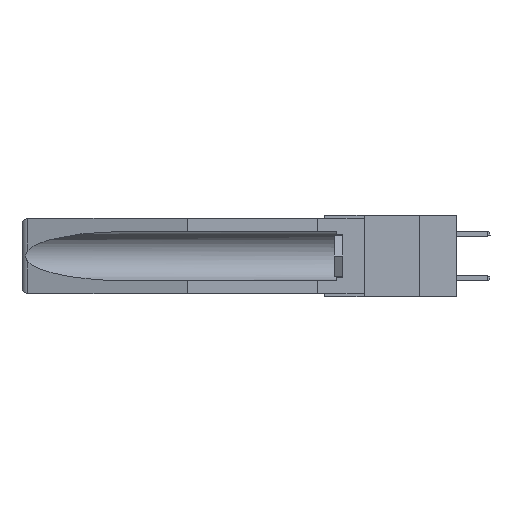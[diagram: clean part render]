
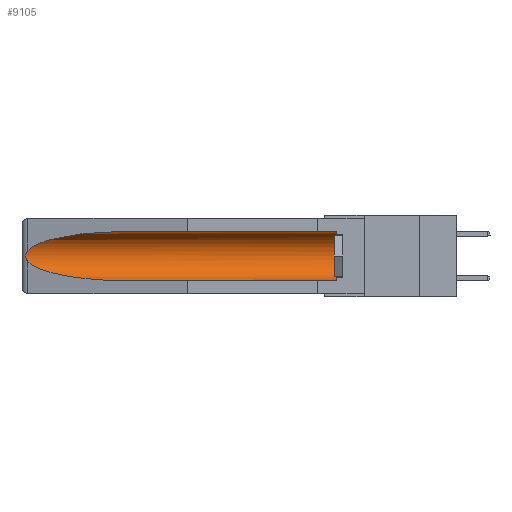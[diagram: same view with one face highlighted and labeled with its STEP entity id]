
A CAD part, left-side view. The second image highlights one B-rep face of the part: STEP entity #9105.
In plain terms, the highlighted cylindrical face has radius 2.857 mm (diameter 5.715 mm), a partial arc.
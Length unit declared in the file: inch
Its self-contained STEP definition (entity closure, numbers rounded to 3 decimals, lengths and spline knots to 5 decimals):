
#644 = DIRECTION ( 'NONE',  ( 0., 1., 0. ) ) ;
#1695 = VERTEX_POINT ( 'NONE', #3598 ) ;
#1882 = CARTESIAN_POINT ( 'NONE',  ( 0.155, 1.07973, -0.284 ) ) ;
#2290 = CARTESIAN_POINT ( 'NONE',  ( 0.155, -0.30754, -0.284 ) ) ;
#2295 = CIRCLE ( 'NONE', #18486, 0.1125 ) ;
#2348 = ORIENTED_EDGE ( 'NONE', *, *, #28603, .T. ) ;
#2690 = ORIENTED_EDGE ( 'NONE', *, *, #3187, .T. ) ;
#2977 = VECTOR ( 'NONE', #13010, 39.37008 ) ;
#3187 = EDGE_CURVE ( 'NONE', #1695, #21045, #13953, .T. ) ;
#3254 = CARTESIAN_POINT ( 'NONE',  ( 0.2673, 1.5327, -0.16383 ) ) ;
#3262 = AXIS2_PLACEMENT_3D ( 'NONE', #29101, #14131, #11287 ) ;
#3360 = CARTESIAN_POINT ( 'NONE',  ( 0.2675, 1.53308, -0.16763 ) ) ;
#3598 = CARTESIAN_POINT ( 'NONE',  ( 0.155, 1.07973, -0.059 ) ) ;
#4143 = CARTESIAN_POINT ( 'NONE',  ( 0.26537, 1.52718, -0.14972 ) ) ;
#5935 = CARTESIAN_POINT ( 'NONE',  ( 0.2675, 1.53308, -0.17534 ) ) ;
#7394 = CARTESIAN_POINT ( 'NONE',  ( 0.155, 0.126, -0.284 ) ) ;
#7539 = CARTESIAN_POINT ( 'NONE',  ( 0.21114, 1.30732, -0.284 ) ) ;
#8003 = CARTESIAN_POINT ( 'NONE',  ( 0.26537, 1.52718, -0.14972 ) ) ;
#8166 = CARTESIAN_POINT ( 'NONE',  ( 0.155, 0.126, -0.059 ) ) ;
#8216 = EDGE_CURVE ( 'NONE', #21045, #9767, #30933, .T. ) ;
#8225 = CARTESIAN_POINT ( 'NONE',  ( 0.26655, 1.53094, -0.18657 ) ) ;
#9105 = ADVANCED_FACE ( 'NONE', ( #24595 ), #30507, .F. ) ;
#9767 = VERTEX_POINT ( 'NONE', #27137 ) ;
#9859 = CARTESIAN_POINT ( 'NONE',  ( 0.25451, 1.48313, -0.24835 ) ) ;
#10286 = VERTEX_POINT ( 'NONE', #1882 ) ;
#10876 = ORIENTED_EDGE ( 'NONE', *, *, #23350, .T. ) ;
#11287 = DIRECTION ( 'NONE',  ( 0., 0., 1. ) ) ;
#11642 = ORIENTED_EDGE ( 'NONE', *, *, #8216, .T. ) ;
#12748 = DIRECTION ( 'NONE',  ( 0., -1., 0. ) ) ;
#12854 = CARTESIAN_POINT ( 'NONE',  ( 0.155, 0.126, -0.1715 ) ) ;
#13010 = DIRECTION ( 'NONE',  ( 0., 1., 0. ) ) ;
#13383 = CARTESIAN_POINT ( 'NONE',  ( 0.26537, 1.52718, -0.19328 ) ) ;
#13953 =( BOUNDED_CURVE ( )  B_SPLINE_CURVE ( 3, ( #27165, #21980, #19331, #19646 ),
 .UNSPECIFIED., .F., .F. ) 
 B_SPLINE_CURVE_WITH_KNOTS ( ( 4, 4 ),
 ( 4.71239, 6.08839 ),
 .UNSPECIFIED. ) 
 CURVE ( )  GEOMETRIC_REPRESENTATION_ITEM ( )  RATIONAL_B_SPLINE_CURVE ( ( 1., 0.848, 0.848, 1. ) ) 
 REPRESENTATION_ITEM ( '' )  );
#14131 = DIRECTION ( 'NONE',  ( 0., 1., 0. ) ) ;
#15490 = CARTESIAN_POINT ( 'NONE',  ( 0.26597, 1.52961, -0.15275 ) ) ;
#17339 = CARTESIAN_POINT ( 'NONE',  ( 0.26537, 1.52718, -0.19328 ) ) ;
#17913 = DIRECTION ( 'NONE',  ( 0., 0., 1. ) ) ;
#18486 = AXIS2_PLACEMENT_3D ( 'NONE', #12854, #12748, #17913 ) ;
#19331 = CARTESIAN_POINT ( 'NONE',  ( 0.25451, 1.48313, -0.09465 ) ) ;
#19614 = ORIENTED_EDGE ( 'NONE', *, *, #22258, .T. ) ;
#19646 = CARTESIAN_POINT ( 'NONE',  ( 0.26537, 1.52718, -0.14972 ) ) ;
#20167 = CARTESIAN_POINT ( 'NONE',  ( 0.155, 1.07973, -0.284 ) ) ;
#20834 = CARTESIAN_POINT ( 'NONE',  ( 0.26597, 1.5296, -0.19026 ) ) ;
#21045 = VERTEX_POINT ( 'NONE', #4143 ) ;
#21980 = CARTESIAN_POINT ( 'NONE',  ( 0.21114, 1.30732, -0.059 ) ) ;
#22258 = EDGE_CURVE ( 'NONE', #29524, #28600, #2295, .T. ) ;
#23350 = EDGE_CURVE ( 'NONE', #9767, #10286, #28496, .T. ) ;
#23442 = CARTESIAN_POINT ( 'NONE',  ( 0.155, -0.30754, -0.059 ) ) ;
#24431 = LINE ( 'NONE', #2290, #27585 ) ;
#24595 = FACE_OUTER_BOUND ( 'NONE', #26365, .T. ) ;
#26365 = EDGE_LOOP ( 'NONE', ( #2690, #11642, #10876, #26623, #19614, #2348 ) ) ;
#26623 = ORIENTED_EDGE ( 'NONE', *, *, #30763, .F. ) ;
#27137 = CARTESIAN_POINT ( 'NONE',  ( 0.26537, 1.52718, -0.19328 ) ) ;
#27165 = CARTESIAN_POINT ( 'NONE',  ( 0.155, 1.07973, -0.059 ) ) ;
#27585 = VECTOR ( 'NONE', #644, 39.37008 ) ;
#28448 = CARTESIAN_POINT ( 'NONE',  ( 0.2673, 1.53269, -0.17917 ) ) ;
#28496 =( BOUNDED_CURVE ( )  B_SPLINE_CURVE ( 3, ( #17339, #9859, #7539, #20167 ),
 .UNSPECIFIED., .F., .T. ) 
 B_SPLINE_CURVE_WITH_KNOTS ( ( 4, 4 ),
 ( 0.1948, 1.5708 ),
 .UNSPECIFIED. ) 
 CURVE ( )  GEOMETRIC_REPRESENTATION_ITEM ( )  RATIONAL_B_SPLINE_CURVE ( ( 1., 0.848, 0.848, 1. ) ) 
 REPRESENTATION_ITEM ( '' )  );
#28600 = VERTEX_POINT ( 'NONE', #8166 ) ;
#28603 = EDGE_CURVE ( 'NONE', #28600, #1695, #29751, .T. ) ;
#29101 = CARTESIAN_POINT ( 'NONE',  ( 0.155, -0.30754, -0.1715 ) ) ;
#29524 = VERTEX_POINT ( 'NONE', #7394 ) ;
#29751 = LINE ( 'NONE', #23442, #2977 ) ;
#30507 = CYLINDRICAL_SURFACE ( 'NONE', #3262, 0.1125 ) ;
#30763 = EDGE_CURVE ( 'NONE', #29524, #10286, #24431, .T. ) ;
#30878 = CARTESIAN_POINT ( 'NONE',  ( 0.26654, 1.53092, -0.15636 ) ) ;
#30933 = B_SPLINE_CURVE_WITH_KNOTS ( 'NONE', 3,
 ( #8003, #15490, #30878, #3254, #3360, #5935, #28448, #8225, #20834, #13383 ),
 .UNSPECIFIED., .F., .F.,
 ( 4, 2, 2, 2, 4 ),
 ( 0., 0.00029, 0.00058, 0.00087, 0.00117 ),
 .UNSPECIFIED. ) ;
